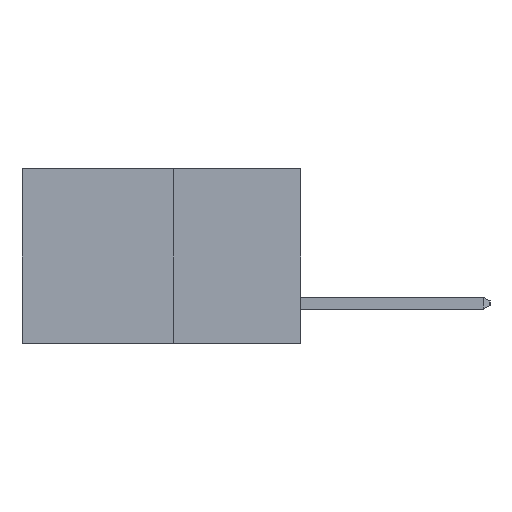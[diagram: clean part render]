
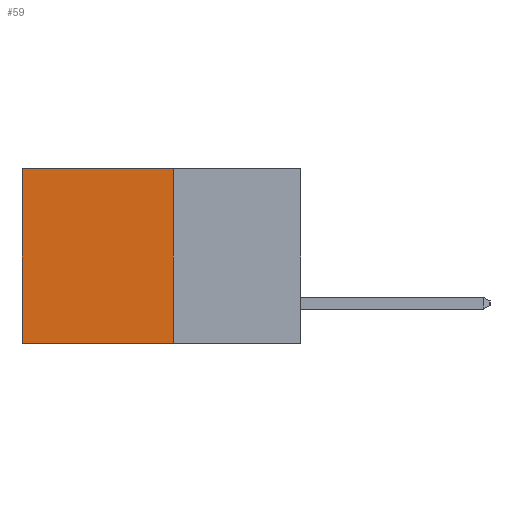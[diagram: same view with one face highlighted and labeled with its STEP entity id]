
A CAD part, left-side view. The second image highlights one B-rep face of the part: STEP entity #59.
In plain terms, the highlighted planar face has unit normal (-1, 0, 0).
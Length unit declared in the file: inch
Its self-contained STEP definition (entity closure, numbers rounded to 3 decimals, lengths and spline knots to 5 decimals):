
#59 = ADVANCED_FACE ( 'NONE', ( #5255 ), #5828, .F. ) ;
#109 = CARTESIAN_POINT ( 'NONE',  ( 0.277, 0.27, -0.37 ) ) ;
#125 = VERTEX_POINT ( 'NONE', #9666 ) ;
#140 = EDGE_LOOP ( 'NONE', ( #8602, #7692, #12613, #2174 ) ) ;
#243 = CARTESIAN_POINT ( 'NONE',  ( 0.277, 0.59, -0.37 ) ) ;
#327 = CARTESIAN_POINT ( 'NONE',  ( 0.277, 0.27, -0.37 ) ) ;
#856 = CARTESIAN_POINT ( 'NONE',  ( 0.277, 0.27, 0. ) ) ;
#1581 = LINE ( 'NONE', #243, #16006 ) ;
#1815 = DIRECTION ( 'NONE',  ( 0., 0., -1. ) ) ;
#2174 = ORIENTED_EDGE ( 'NONE', *, *, #2816, .T. ) ;
#2816 = EDGE_CURVE ( 'NONE', #125, #9842, #16137, .T. ) ;
#3164 = CARTESIAN_POINT ( 'NONE',  ( 0.277, 0.27, -0.37 ) ) ;
#3736 = VECTOR ( 'NONE', #1815, 39.37008 ) ;
#5138 = EDGE_CURVE ( 'NONE', #125, #13579, #7904, .T. ) ;
#5255 = FACE_OUTER_BOUND ( 'NONE', #140, .T. ) ;
#5621 = LINE ( 'NONE', #11968, #17427 ) ;
#5828 = PLANE ( 'NONE',  #14847 ) ;
#6660 = EDGE_CURVE ( 'NONE', #9842, #8826, #1581, .T. ) ;
#7692 = ORIENTED_EDGE ( 'NONE', *, *, #8792, .F. ) ;
#7710 = DIRECTION ( 'NONE',  ( 0., 1., 0. ) ) ;
#7904 = LINE ( 'NONE', #327, #3736 ) ;
#8602 = ORIENTED_EDGE ( 'NONE', *, *, #6660, .T. ) ;
#8792 = EDGE_CURVE ( 'NONE', #13579, #8826, #5621, .T. ) ;
#8826 = VERTEX_POINT ( 'NONE', #17407 ) ;
#9666 = CARTESIAN_POINT ( 'NONE',  ( 0.277, 0.27, 0. ) ) ;
#9842 = VERTEX_POINT ( 'NONE', #9947 ) ;
#9947 = CARTESIAN_POINT ( 'NONE',  ( 0.277, 0.59, 0. ) ) ;
#10842 = DIRECTION ( 'NONE',  ( 0., 1., 0. ) ) ;
#11435 = DIRECTION ( 'NONE',  ( 0., 0., -1. ) ) ;
#11968 = CARTESIAN_POINT ( 'NONE',  ( 0.277, 0.27, -0.37 ) ) ;
#12613 = ORIENTED_EDGE ( 'NONE', *, *, #5138, .F. ) ;
#13579 = VERTEX_POINT ( 'NONE', #109 ) ;
#14402 = DIRECTION ( 'NONE',  ( 0., 0., -1. ) ) ;
#14847 = AXIS2_PLACEMENT_3D ( 'NONE', #3164, #17109, #11435 ) ;
#15732 = VECTOR ( 'NONE', #10842, 39.37008 ) ;
#16006 = VECTOR ( 'NONE', #14402, 39.37008 ) ;
#16137 = LINE ( 'NONE', #856, #15732 ) ;
#17109 = DIRECTION ( 'NONE',  ( 1., 0., 0. ) ) ;
#17407 = CARTESIAN_POINT ( 'NONE',  ( 0.277, 0.59, -0.37 ) ) ;
#17427 = VECTOR ( 'NONE', #7710, 39.37008 ) ;
